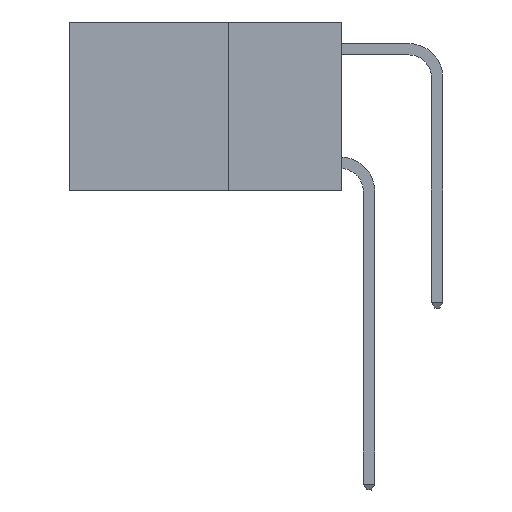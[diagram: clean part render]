
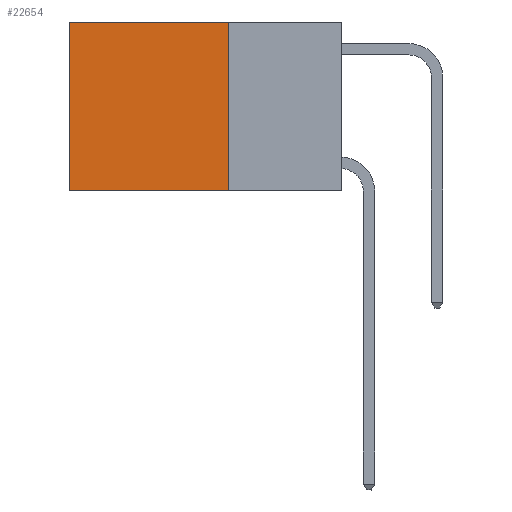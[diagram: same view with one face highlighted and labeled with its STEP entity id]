
A CAD part, left-side view. The second image highlights one B-rep face of the part: STEP entity #22654.
In plain terms, the highlighted planar face has unit normal (-1, 0, 0).
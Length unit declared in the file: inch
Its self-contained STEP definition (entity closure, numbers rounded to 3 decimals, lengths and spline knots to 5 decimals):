
#141 = CARTESIAN_POINT ( 'NONE',  ( 0.2625, 0.25, -0.37 ) ) ;
#497 = DIRECTION ( 'NONE',  ( 0., 0., -1. ) ) ;
#752 = VECTOR ( 'NONE', #3325, 39.37008 ) ;
#2443 = CARTESIAN_POINT ( 'NONE',  ( 0.2625, 0.25, 0. ) ) ;
#2786 = CARTESIAN_POINT ( 'NONE',  ( 0.2625, 0.6, 0. ) ) ;
#3195 = DIRECTION ( 'NONE',  ( 0., 1., 0. ) ) ;
#3325 = DIRECTION ( 'NONE',  ( 0., 0., -1. ) ) ;
#3887 = EDGE_CURVE ( 'NONE', #14809, #15684, #12756, .T. ) ;
#5503 = AXIS2_PLACEMENT_3D ( 'NONE', #18210, #16141, #18305 ) ;
#7624 = EDGE_CURVE ( 'NONE', #17229, #14809, #25213, .T. ) ;
#8593 = DIRECTION ( 'NONE',  ( 0., 1., 0. ) ) ;
#9040 = EDGE_LOOP ( 'NONE', ( #16336, #25414, #26619, #14778 ) ) ;
#9398 = LINE ( 'NONE', #141, #21152 ) ;
#9535 = CARTESIAN_POINT ( 'NONE',  ( 0.2625, 0.25, 0. ) ) ;
#12756 = LINE ( 'NONE', #2786, #752 ) ;
#14778 = ORIENTED_EDGE ( 'NONE', *, *, #7624, .T. ) ;
#14809 = VERTEX_POINT ( 'NONE', #26995 ) ;
#15684 = VERTEX_POINT ( 'NONE', #26093 ) ;
#16076 = CARTESIAN_POINT ( 'NONE',  ( 0.2625, 0.25, -0.37 ) ) ;
#16141 = DIRECTION ( 'NONE',  ( 1., 0., 0. ) ) ;
#16336 = ORIENTED_EDGE ( 'NONE', *, *, #3887, .T. ) ;
#17229 = VERTEX_POINT ( 'NONE', #9535 ) ;
#18210 = CARTESIAN_POINT ( 'NONE',  ( 0.2625, 0.25, 0. ) ) ;
#18305 = DIRECTION ( 'NONE',  ( 0., 0., -1. ) ) ;
#20202 = VECTOR ( 'NONE', #3195, 39.37008 ) ;
#20617 = VECTOR ( 'NONE', #497, 39.37008 ) ;
#21152 = VECTOR ( 'NONE', #8593, 39.37008 ) ;
#21338 = EDGE_CURVE ( 'NONE', #23046, #15684, #9398, .T. ) ;
#21387 = CARTESIAN_POINT ( 'NONE',  ( 0.2625, 0.25, 0. ) ) ;
#22441 = FACE_OUTER_BOUND ( 'NONE', #9040, .T. ) ;
#22654 = ADVANCED_FACE ( 'NONE', ( #22441 ), #24567, .F. ) ;
#23046 = VERTEX_POINT ( 'NONE', #16076 ) ;
#24270 = LINE ( 'NONE', #21387, #20617 ) ;
#24567 = PLANE ( 'NONE',  #5503 ) ;
#25213 = LINE ( 'NONE', #2443, #20202 ) ;
#25414 = ORIENTED_EDGE ( 'NONE', *, *, #21338, .F. ) ;
#26093 = CARTESIAN_POINT ( 'NONE',  ( 0.2625, 0.6, -0.37 ) ) ;
#26619 = ORIENTED_EDGE ( 'NONE', *, *, #27300, .F. ) ;
#26995 = CARTESIAN_POINT ( 'NONE',  ( 0.2625, 0.6, 0. ) ) ;
#27300 = EDGE_CURVE ( 'NONE', #17229, #23046, #24270, .T. ) ;
